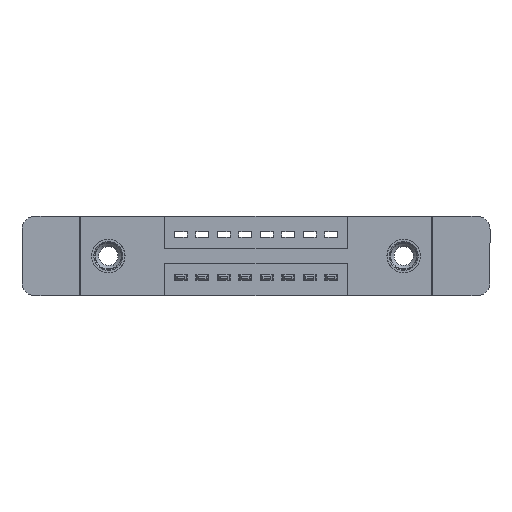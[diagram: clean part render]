
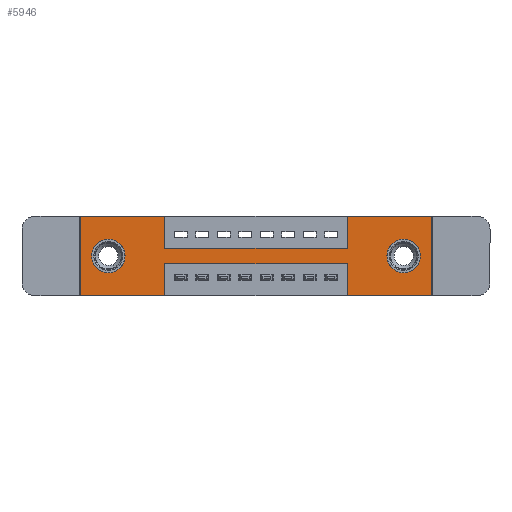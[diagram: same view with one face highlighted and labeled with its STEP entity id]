
A CAD part, front view. The second image highlights one B-rep face of the part: STEP entity #5946.
In plain terms, the highlighted planar face has unit normal (0, -1, 0).
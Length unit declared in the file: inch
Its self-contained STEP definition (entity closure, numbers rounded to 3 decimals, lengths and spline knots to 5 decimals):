
#16 = LINE ( 'NONE', #4443, #8107 ) ;
#31 = LINE ( 'NONE', #12363, #7930 ) ;
#248 = DIRECTION ( 'NONE',  ( 0., 1., 0. ) ) ;
#334 = ORIENTED_EDGE ( 'NONE', *, *, #11960, .F. ) ;
#378 = ORIENTED_EDGE ( 'NONE', *, *, #8363, .F. ) ;
#400 = CARTESIAN_POINT ( 'NONE',  ( 0.13, 0., -0.107 ) ) ;
#482 = CARTESIAN_POINT ( 'NONE',  ( 1.505, 0., -0.185 ) ) ;
#685 = DIRECTION ( 'NONE',  ( 0., 0., 1. ) ) ;
#793 = EDGE_CURVE ( 'NONE', #5221, #11050, #31, .T. ) ;
#830 = CARTESIAN_POINT ( 'NONE',  ( 0.13, 0., -0.263 ) ) ;
#972 = CARTESIAN_POINT ( 'NONE',  ( 1.2425, 0., 0. ) ) ;
#982 = EDGE_CURVE ( 'NONE', #13852, #6389, #16, .T. ) ;
#1006 = FACE_BOUND ( 'NONE', #6502, .T. ) ;
#1024 = CARTESIAN_POINT ( 'NONE',  ( 0.3925, 0., -0.37 ) ) ;
#1437 = VECTOR ( 'NONE', #7329, 39.37008 ) ;
#1748 = DIRECTION ( 'NONE',  ( 0., 0., -1. ) ) ;
#1850 = CARTESIAN_POINT ( 'NONE',  ( 0., 0., 0. ) ) ;
#2153 = EDGE_CURVE ( 'NONE', #4433, #11113, #7681, .T. ) ;
#2586 = CARTESIAN_POINT ( 'NONE',  ( 0., 0., 0. ) ) ;
#2780 = CIRCLE ( 'NONE', #3646, 0.078 ) ;
#2873 = AXIS2_PLACEMENT_3D ( 'NONE', #10100, #7711, #1748 ) ;
#2925 = EDGE_CURVE ( 'NONE', #15500, #5221, #7474, .T. ) ;
#3060 = CARTESIAN_POINT ( 'NONE',  ( 1.2425, 0., -0.15 ) ) ;
#3103 = DIRECTION ( 'NONE',  ( 0., 1., 0. ) ) ;
#3147 = VERTEX_POINT ( 'NONE', #10722 ) ;
#3349 = VECTOR ( 'NONE', #6405, 39.37008 ) ;
#3352 = EDGE_CURVE ( 'NONE', #14584, #15125, #5783, .T. ) ;
#3450 = EDGE_CURVE ( 'NONE', #15125, #13702, #6127, .T. ) ;
#3646 = AXIS2_PLACEMENT_3D ( 'NONE', #13731, #248, #12899 ) ;
#3920 = ORIENTED_EDGE ( 'NONE', *, *, #9169, .T. ) ;
#4089 = ORIENTED_EDGE ( 'NONE', *, *, #2153, .F. ) ;
#4131 = EDGE_CURVE ( 'NONE', #6389, #15115, #8926, .T. ) ;
#4141 = DIRECTION ( 'NONE',  ( 0., 0., 1. ) ) ;
#4288 = VECTOR ( 'NONE', #7410, 39.37008 ) ;
#4433 = VERTEX_POINT ( 'NONE', #8125 ) ;
#4443 = CARTESIAN_POINT ( 'NONE',  ( 1.2425, 0., -0.37 ) ) ;
#4688 = VECTOR ( 'NONE', #7842, 39.37008 ) ;
#4714 = CARTESIAN_POINT ( 'NONE',  ( 0.13, 0., -0.185 ) ) ;
#4930 = FACE_OUTER_BOUND ( 'NONE', #9519, .T. ) ;
#5042 = ORIENTED_EDGE ( 'NONE', *, *, #14093, .F. ) ;
#5044 = EDGE_LOOP ( 'NONE', ( #14634, #3920 ) ) ;
#5095 = CARTESIAN_POINT ( 'NONE',  ( 1.635, 0., 0. ) ) ;
#5145 = DIRECTION ( 'NONE',  ( 0., 0., -1. ) ) ;
#5221 = VERTEX_POINT ( 'NONE', #14530 ) ;
#5317 = LINE ( 'NONE', #1024, #14156 ) ;
#5475 = ORIENTED_EDGE ( 'NONE', *, *, #3352, .F. ) ;
#5587 = VERTEX_POINT ( 'NONE', #830 ) ;
#5658 = EDGE_CURVE ( 'NONE', #12107, #5587, #8322, .T. ) ;
#5680 = DIRECTION ( 'NONE',  ( 1., 0., 0. ) ) ;
#5693 = FACE_BOUND ( 'NONE', #5044, .T. ) ;
#5694 = LINE ( 'NONE', #13983, #7753 ) ;
#5783 = LINE ( 'NONE', #2586, #4288 ) ;
#5901 = DIRECTION ( 'NONE',  ( 0., 1., 0. ) ) ;
#5903 = VECTOR ( 'NONE', #13394, 39.37008 ) ;
#5946 = ADVANCED_FACE ( 'NONE', ( #1006, #5693, #4930 ), #8860, .T. ) ;
#6127 = LINE ( 'NONE', #5095, #3349 ) ;
#6225 = AXIS2_PLACEMENT_3D ( 'NONE', #482, #13545, #5145 ) ;
#6389 = VERTEX_POINT ( 'NONE', #11012 ) ;
#6405 = DIRECTION ( 'NONE',  ( 0., 0., -1. ) ) ;
#6502 = EDGE_LOOP ( 'NONE', ( #14913, #7649 ) ) ;
#6867 = LINE ( 'NONE', #972, #12114 ) ;
#7102 = DIRECTION ( 'NONE',  ( 0., 0., -1. ) ) ;
#7240 = CARTESIAN_POINT ( 'NONE',  ( 0.3925, 0., -0.22 ) ) ;
#7280 = ORIENTED_EDGE ( 'NONE', *, *, #982, .F. ) ;
#7329 = DIRECTION ( 'NONE',  ( -1., 0., 0. ) ) ;
#7357 = DIRECTION ( 'NONE',  ( 0., 0., 1. ) ) ;
#7410 = DIRECTION ( 'NONE',  ( 1., 0., 0. ) ) ;
#7474 = LINE ( 'NONE', #14917, #12736 ) ;
#7649 = ORIENTED_EDGE ( 'NONE', *, *, #12247, .T. ) ;
#7681 = LINE ( 'NONE', #14795, #12563 ) ;
#7682 = DIRECTION ( 'NONE',  ( -1., 0., 0. ) ) ;
#7711 = DIRECTION ( 'NONE',  ( 0., -1., 0. ) ) ;
#7753 = VECTOR ( 'NONE', #5680, 39.37008 ) ;
#7842 = DIRECTION ( 'NONE',  ( 0., 0., -1. ) ) ;
#7930 = VECTOR ( 'NONE', #4141, 39.37008 ) ;
#8053 = DIRECTION ( 'NONE',  ( 0., 0., 1. ) ) ;
#8107 = VECTOR ( 'NONE', #14264, 39.37008 ) ;
#8125 = CARTESIAN_POINT ( 'NONE',  ( 0.3925, 0., -0.15 ) ) ;
#8217 = AXIS2_PLACEMENT_3D ( 'NONE', #15507, #3103, #685 ) ;
#8284 = CARTESIAN_POINT ( 'NONE',  ( 1.2425, 0., 0. ) ) ;
#8292 = AXIS2_PLACEMENT_3D ( 'NONE', #4714, #5901, #7357 ) ;
#8322 = CIRCLE ( 'NONE', #8292, 0.078 ) ;
#8363 = EDGE_CURVE ( 'NONE', #11050, #10517, #5694, .T. ) ;
#8860 = PLANE ( 'NONE',  #2873 ) ;
#8926 = LINE ( 'NONE', #7240, #1437 ) ;
#9052 = CARTESIAN_POINT ( 'NONE',  ( 0.3925, 0., 0. ) ) ;
#9169 = EDGE_CURVE ( 'NONE', #5587, #12107, #15505, .T. ) ;
#9519 = EDGE_LOOP ( 'NONE', ( #12796, #14067, #7280, #5042, #14936, #5475, #13136, #4089, #334, #378, #10757, #11573 ) ) ;
#9540 = CARTESIAN_POINT ( 'NONE',  ( 1.505, 0., -0.263 ) ) ;
#10100 = CARTESIAN_POINT ( 'NONE',  ( 0., 0., -0.37 ) ) ;
#10162 = CARTESIAN_POINT ( 'NONE',  ( 1.635, 0., -0.37 ) ) ;
#10425 = CIRCLE ( 'NONE', #6225, 0.078 ) ;
#10494 = LINE ( 'NONE', #15077, #4688 ) ;
#10517 = VERTEX_POINT ( 'NONE', #9052 ) ;
#10722 = CARTESIAN_POINT ( 'NONE',  ( 1.505, 0., -0.107 ) ) ;
#10757 = ORIENTED_EDGE ( 'NONE', *, *, #793, .F. ) ;
#10898 = VERTEX_POINT ( 'NONE', #9540 ) ;
#11012 = CARTESIAN_POINT ( 'NONE',  ( 1.2425, 0., -0.22 ) ) ;
#11050 = VERTEX_POINT ( 'NONE', #1850 ) ;
#11096 = CARTESIAN_POINT ( 'NONE',  ( 0.3925, 0., -0.22 ) ) ;
#11113 = VERTEX_POINT ( 'NONE', #3060 ) ;
#11562 = CARTESIAN_POINT ( 'NONE',  ( 1.2425, 0., -0.37 ) ) ;
#11573 = ORIENTED_EDGE ( 'NONE', *, *, #2925, .F. ) ;
#11960 = EDGE_CURVE ( 'NONE', #10517, #4433, #10494, .T. ) ;
#12107 = VERTEX_POINT ( 'NONE', #400 ) ;
#12114 = VECTOR ( 'NONE', #8053, 39.37008 ) ;
#12247 = EDGE_CURVE ( 'NONE', #10898, #3147, #2780, .T. ) ;
#12363 = CARTESIAN_POINT ( 'NONE',  ( 0., 0., 0. ) ) ;
#12563 = VECTOR ( 'NONE', #13461, 39.37008 ) ;
#12736 = VECTOR ( 'NONE', #7682, 39.37008 ) ;
#12796 = ORIENTED_EDGE ( 'NONE', *, *, #13907, .F. ) ;
#12899 = DIRECTION ( 'NONE',  ( 0., 0., -1. ) ) ;
#13112 = CARTESIAN_POINT ( 'NONE',  ( 0.3925, 0., -0.37 ) ) ;
#13136 = ORIENTED_EDGE ( 'NONE', *, *, #13797, .F. ) ;
#13233 = LINE ( 'NONE', #13237, #5903 ) ;
#13237 = CARTESIAN_POINT ( 'NONE',  ( 0., 0., -0.37 ) ) ;
#13394 = DIRECTION ( 'NONE',  ( -1., 0., 0. ) ) ;
#13461 = DIRECTION ( 'NONE',  ( 1., 0., 0. ) ) ;
#13545 = DIRECTION ( 'NONE',  ( 0., 1., 0. ) ) ;
#13702 = VERTEX_POINT ( 'NONE', #10162 ) ;
#13731 = CARTESIAN_POINT ( 'NONE',  ( 1.505, 0., -0.185 ) ) ;
#13797 = EDGE_CURVE ( 'NONE', #11113, #14584, #6867, .T. ) ;
#13852 = VERTEX_POINT ( 'NONE', #11562 ) ;
#13907 = EDGE_CURVE ( 'NONE', #15115, #15500, #5317, .T. ) ;
#13983 = CARTESIAN_POINT ( 'NONE',  ( 0., 0., 0. ) ) ;
#14067 = ORIENTED_EDGE ( 'NONE', *, *, #4131, .F. ) ;
#14093 = EDGE_CURVE ( 'NONE', #13702, #13852, #13233, .T. ) ;
#14156 = VECTOR ( 'NONE', #7102, 39.37008 ) ;
#14172 = EDGE_CURVE ( 'NONE', #3147, #10898, #10425, .T. ) ;
#14264 = DIRECTION ( 'NONE',  ( 0., 0., 1. ) ) ;
#14530 = CARTESIAN_POINT ( 'NONE',  ( 0., 0., -0.37 ) ) ;
#14584 = VERTEX_POINT ( 'NONE', #8284 ) ;
#14634 = ORIENTED_EDGE ( 'NONE', *, *, #5658, .T. ) ;
#14702 = CARTESIAN_POINT ( 'NONE',  ( 1.635, 0., 0. ) ) ;
#14795 = CARTESIAN_POINT ( 'NONE',  ( 0.3925, 0., -0.15 ) ) ;
#14913 = ORIENTED_EDGE ( 'NONE', *, *, #14172, .T. ) ;
#14917 = CARTESIAN_POINT ( 'NONE',  ( 0., 0., -0.37 ) ) ;
#14936 = ORIENTED_EDGE ( 'NONE', *, *, #3450, .F. ) ;
#15077 = CARTESIAN_POINT ( 'NONE',  ( 0.3925, 0., 0. ) ) ;
#15115 = VERTEX_POINT ( 'NONE', #11096 ) ;
#15125 = VERTEX_POINT ( 'NONE', #14702 ) ;
#15500 = VERTEX_POINT ( 'NONE', #13112 ) ;
#15505 = CIRCLE ( 'NONE', #8217, 0.078 ) ;
#15507 = CARTESIAN_POINT ( 'NONE',  ( 0.13, 0., -0.185 ) ) ;
